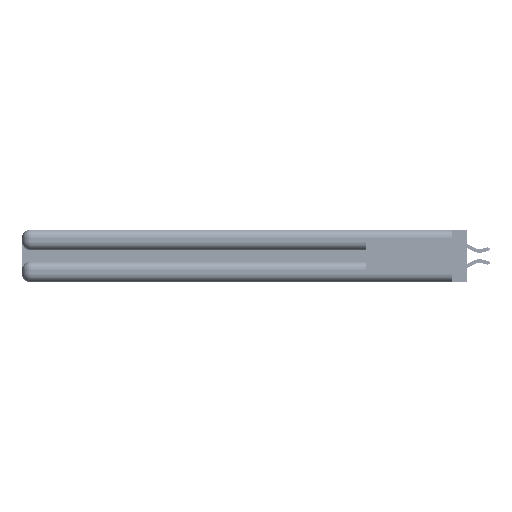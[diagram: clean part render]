
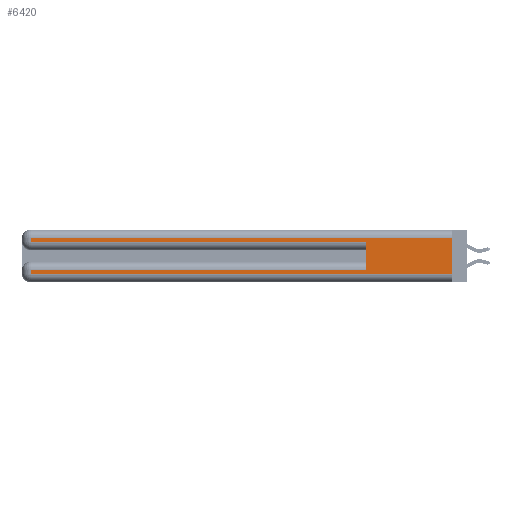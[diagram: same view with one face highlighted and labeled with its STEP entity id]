
A CAD part, left-side view. The second image highlights one B-rep face of the part: STEP entity #6420.
In plain terms, the highlighted planar face has unit normal (-1, 0, 0).
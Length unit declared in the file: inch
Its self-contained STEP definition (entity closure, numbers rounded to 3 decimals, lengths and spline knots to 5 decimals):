
#2491 = LINE ( 'NONE', #51297, #22135 ) ;
#2832 = DIRECTION ( 'NONE',  ( 0., 0., -1. ) ) ;
#4001 = AXIS2_PLACEMENT_3D ( 'NONE', #33949, #11678, #7188 ) ;
#4855 = VERTEX_POINT ( 'NONE', #8180 ) ;
#5629 = EDGE_LOOP ( 'NONE', ( #49286, #40029, #30394, #11376, #20104, #36028, #32732, #34485 ) ) ;
#5938 = VERTEX_POINT ( 'NONE', #25103 ) ;
#6420 = ADVANCED_FACE ( 'NONE', ( #9051 ), #34380, .F. ) ;
#6978 = CARTESIAN_POINT ( 'NONE',  ( 0., 2.94, 0.31 ) ) ;
#7188 = DIRECTION ( 'NONE',  ( 0., 0., -1. ) ) ;
#7534 = VECTOR ( 'NONE', #51664, 39.37008 ) ;
#7866 = EDGE_CURVE ( 'NONE', #18175, #22661, #14072, .T. ) ;
#8180 = CARTESIAN_POINT ( 'NONE',  ( 0., 0., 0.06 ) ) ;
#8248 = VERTEX_POINT ( 'NONE', #29467 ) ;
#8668 = DIRECTION ( 'NONE',  ( 0., 0., -1. ) ) ;
#9051 = FACE_OUTER_BOUND ( 'NONE', #5629, .T. ) ;
#10056 = EDGE_CURVE ( 'NONE', #40096, #4855, #20404, .T. ) ;
#11111 = CARTESIAN_POINT ( 'NONE',  ( 0., 2.94, 0.37 ) ) ;
#11376 = ORIENTED_EDGE ( 'NONE', *, *, #7866, .T. ) ;
#11539 = LINE ( 'NONE', #22483, #18754 ) ;
#11678 = DIRECTION ( 'NONE',  ( 1., 0., 0. ) ) ;
#12156 = CARTESIAN_POINT ( 'NONE',  ( 0., 2.94, 0.285 ) ) ;
#13323 = EDGE_CURVE ( 'NONE', #5938, #22661, #41207, .T. ) ;
#13867 = DIRECTION ( 'NONE',  ( 0., 1., 0. ) ) ;
#14072 = LINE ( 'NONE', #39414, #7534 ) ;
#14873 = EDGE_CURVE ( 'NONE', #40096, #47703, #2491, .T. ) ;
#17402 = LINE ( 'NONE', #25798, #41512 ) ;
#18175 = VERTEX_POINT ( 'NONE', #12156 ) ;
#18754 = VECTOR ( 'NONE', #13867, 39.37008 ) ;
#20104 = ORIENTED_EDGE ( 'NONE', *, *, #13323, .F. ) ;
#20252 = EDGE_CURVE ( 'NONE', #36419, #8248, #32701, .T. ) ;
#20404 = LINE ( 'NONE', #48165, #34721 ) ;
#20707 = CARTESIAN_POINT ( 'NONE',  ( 0., 0.6, 0.145 ) ) ;
#22135 = VECTOR ( 'NONE', #32264, 39.37008 ) ;
#22483 = CARTESIAN_POINT ( 'NONE',  ( 0., 0., 0.085 ) ) ;
#22661 = VERTEX_POINT ( 'NONE', #50738 ) ;
#25103 = CARTESIAN_POINT ( 'NONE',  ( 0., 0.6, 0.085 ) ) ;
#25798 = CARTESIAN_POINT ( 'NONE',  ( 0., 0., 0.06 ) ) ;
#26881 = VECTOR ( 'NONE', #8668, 39.37008 ) ;
#28144 = CARTESIAN_POINT ( 'NONE',  ( 0., 0., 0.31 ) ) ;
#28627 = EDGE_CURVE ( 'NONE', #47703, #18175, #41239, .T. ) ;
#29467 = CARTESIAN_POINT ( 'NONE',  ( 0., 2.94, 0.06 ) ) ;
#30143 = VECTOR ( 'NONE', #44515, 39.37008 ) ;
#30394 = ORIENTED_EDGE ( 'NONE', *, *, #28627, .T. ) ;
#32264 = DIRECTION ( 'NONE',  ( 0., 1., 0. ) ) ;
#32701 = LINE ( 'NONE', #46428, #26881 ) ;
#32732 = ORIENTED_EDGE ( 'NONE', *, *, #20252, .T. ) ;
#33949 = CARTESIAN_POINT ( 'NONE',  ( 0., 0., 0.37 ) ) ;
#34000 = VECTOR ( 'NONE', #45685, 39.37008 ) ;
#34380 = PLANE ( 'NONE',  #4001 ) ;
#34485 = ORIENTED_EDGE ( 'NONE', *, *, #44075, .T. ) ;
#34721 = VECTOR ( 'NONE', #2832, 39.37008 ) ;
#36028 = ORIENTED_EDGE ( 'NONE', *, *, #42819, .T. ) ;
#36419 = VERTEX_POINT ( 'NONE', #41188 ) ;
#39414 = CARTESIAN_POINT ( 'NONE',  ( 0., 0., 0.285 ) ) ;
#40029 = ORIENTED_EDGE ( 'NONE', *, *, #14873, .T. ) ;
#40096 = VERTEX_POINT ( 'NONE', #28144 ) ;
#41188 = CARTESIAN_POINT ( 'NONE',  ( 0., 2.94, 0.085 ) ) ;
#41207 = LINE ( 'NONE', #20707, #34000 ) ;
#41239 = LINE ( 'NONE', #11111, #30143 ) ;
#41512 = VECTOR ( 'NONE', #42546, 39.37008 ) ;
#42546 = DIRECTION ( 'NONE',  ( 0., -1., 0. ) ) ;
#42819 = EDGE_CURVE ( 'NONE', #5938, #36419, #11539, .T. ) ;
#44075 = EDGE_CURVE ( 'NONE', #8248, #4855, #17402, .T. ) ;
#44515 = DIRECTION ( 'NONE',  ( 0., 0., -1. ) ) ;
#45685 = DIRECTION ( 'NONE',  ( 0., 0., 1. ) ) ;
#46428 = CARTESIAN_POINT ( 'NONE',  ( 0., 2.94, 0.37 ) ) ;
#47703 = VERTEX_POINT ( 'NONE', #6978 ) ;
#48165 = CARTESIAN_POINT ( 'NONE',  ( 0., 0., 0.37 ) ) ;
#49286 = ORIENTED_EDGE ( 'NONE', *, *, #10056, .F. ) ;
#50738 = CARTESIAN_POINT ( 'NONE',  ( 0., 0.6, 0.285 ) ) ;
#51297 = CARTESIAN_POINT ( 'NONE',  ( 0., 0., 0.31 ) ) ;
#51664 = DIRECTION ( 'NONE',  ( 0., -1., 0. ) ) ;
